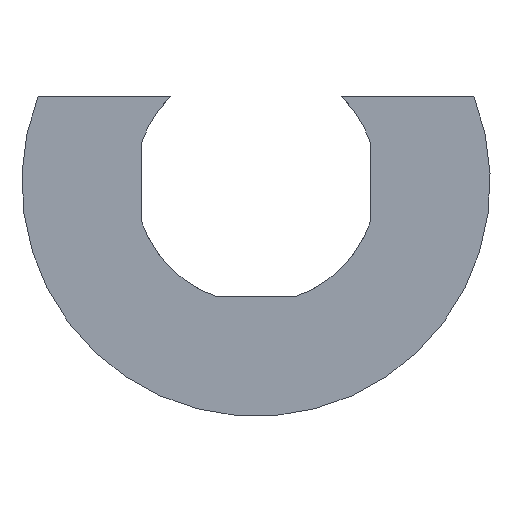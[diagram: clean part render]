
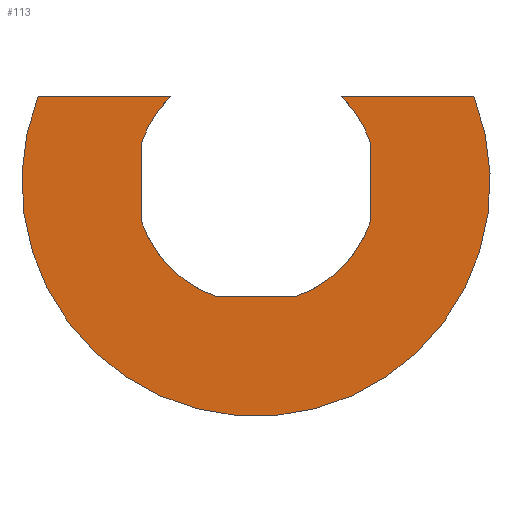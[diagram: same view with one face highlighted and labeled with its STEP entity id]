
A CAD part, front view. The second image highlights one B-rep face of the part: STEP entity #113.
In plain terms, the highlighted planar face has unit normal (0, -1, 0).
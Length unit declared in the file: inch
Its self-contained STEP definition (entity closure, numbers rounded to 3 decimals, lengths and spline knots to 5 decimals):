
#43 = EDGE_CURVE ( 'NONE', #423, #445, #149, .T. ) ;
#46 = EDGE_CURVE ( 'NONE', #447, #430, #778, .T. ) ;
#50 = EDGE_CURVE ( 'NONE', #438, #419, #141, .T. ) ;
#54 = EDGE_CURVE ( 'NONE', #419, #403, #821, .T. ) ;
#57 = EDGE_CURVE ( 'NONE', #418, #423, #824, .T. ) ;
#62 = EDGE_CURVE ( 'NONE', #447, #446, #145, .T. ) ;
#67 = EDGE_CURVE ( 'NONE', #446, #438, #838, .T. ) ;
#68 = EDGE_CURVE ( 'NONE', #418, #430, #143, .T. ) ;
#69 = EDGE_CURVE ( 'NONE', #405, #445, #840, .T. ) ;
#71 = EDGE_CURVE ( 'NONE', #403, #405, #168, .T. ) ;
#113 = ADVANCED_FACE ( 'NONE', ( #332 ), #987, .F. ) ;
#141 = CIRCLE ( 'NONE', #268, 0.60076 ) ;
#143 = CIRCLE ( 'NONE', #255, 0.60076 ) ;
#145 = CIRCLE ( 'NONE', #258, 0.60076 ) ;
#149 = CIRCLE ( 'NONE', #243, 1.16129 ) ;
#168 = CIRCLE ( 'NONE', #259, 0.60076 ) ;
#243 = AXIS2_PLACEMENT_3D ( 'NONE', #771, #768, #783 ) ;
#250 = VECTOR ( 'NONE', #859, 39.37008 ) ;
#255 = AXIS2_PLACEMENT_3D ( 'NONE', #846, #835, #832 ) ;
#256 = VECTOR ( 'NONE', #825, 39.37008 ) ;
#257 = VECTOR ( 'NONE', #806, 39.37008 ) ;
#258 = AXIS2_PLACEMENT_3D ( 'NONE', #815, #833, #850 ) ;
#259 = AXIS2_PLACEMENT_3D ( 'NONE', #851, #836, #853 ) ;
#260 = VECTOR ( 'NONE', #779, 39.37008 ) ;
#268 = AXIS2_PLACEMENT_3D ( 'NONE', #794, #787, #793 ) ;
#288 = VECTOR ( 'NONE', #852, 39.37008 ) ;
#310 = AXIS2_PLACEMENT_3D ( 'NONE', #990, #960, #963 ) ;
#332 = FACE_OUTER_BOUND ( 'NONE', #477, .T. ) ;
#403 = VERTEX_POINT ( 'NONE', #1159 ) ;
#405 = VERTEX_POINT ( 'NONE', #1160 ) ;
#418 = VERTEX_POINT ( 'NONE', #1179 ) ;
#419 = VERTEX_POINT ( 'NONE', #1184 ) ;
#423 = VERTEX_POINT ( 'NONE', #1183 ) ;
#430 = VERTEX_POINT ( 'NONE', #1098 ) ;
#438 = VERTEX_POINT ( 'NONE', #1097 ) ;
#445 = VERTEX_POINT ( 'NONE', #1048 ) ;
#446 = VERTEX_POINT ( 'NONE', #1050 ) ;
#447 = VERTEX_POINT ( 'NONE', #1033 ) ;
#477 = EDGE_LOOP ( 'NONE', ( #531, #543, #535, #525, #521, #522, #536, #542, #530, #519 ) ) ;
#519 = ORIENTED_EDGE ( 'NONE', *, *, #54, .T. ) ;
#521 = ORIENTED_EDGE ( 'NONE', *, *, #68, .T. ) ;
#522 = ORIENTED_EDGE ( 'NONE', *, *, #46, .F. ) ;
#525 = ORIENTED_EDGE ( 'NONE', *, *, #57, .F. ) ;
#530 = ORIENTED_EDGE ( 'NONE', *, *, #50, .T. ) ;
#531 = ORIENTED_EDGE ( 'NONE', *, *, #71, .T. ) ;
#535 = ORIENTED_EDGE ( 'NONE', *, *, #43, .F. ) ;
#536 = ORIENTED_EDGE ( 'NONE', *, *, #62, .T. ) ;
#542 = ORIENTED_EDGE ( 'NONE', *, *, #67, .T. ) ;
#543 = ORIENTED_EDGE ( 'NONE', *, *, #69, .T. ) ;
#768 = DIRECTION ( 'NONE',  ( 0., 1., 0. ) ) ;
#771 = CARTESIAN_POINT ( 'NONE',  ( -0.56759, 0., -0.19685 ) ) ;
#778 = LINE ( 'NONE', #786, #260 ) ;
#779 = DIRECTION ( 'NONE',  ( 0., 0., 1. ) ) ;
#783 = DIRECTION ( 'NONE',  ( 0., 0., 1. ) ) ;
#786 = CARTESIAN_POINT ( 'NONE',  ( 0., 0., 0. ) ) ;
#787 = DIRECTION ( 'NONE',  ( 0., 1., 0. ) ) ;
#793 = DIRECTION ( 'NONE',  ( 0., 0., 1. ) ) ;
#794 = CARTESIAN_POINT ( 'NONE',  ( -0.56759, 0., -0.19685 ) ) ;
#806 = DIRECTION ( 'NONE',  ( 0., 0., 1. ) ) ;
#807 = CARTESIAN_POINT ( 'NONE',  ( -1.13518, 0., 0. ) ) ;
#809 = CARTESIAN_POINT ( 'NONE',  ( 0., 0., 0.22795 ) ) ;
#815 = CARTESIAN_POINT ( 'NONE',  ( -0.56759, 0., -0.19685 ) ) ;
#821 = LINE ( 'NONE', #807, #257 ) ;
#824 = LINE ( 'NONE', #809, #256 ) ;
#825 = DIRECTION ( 'NONE',  ( 1., 0., 0. ) ) ;
#832 = DIRECTION ( 'NONE',  ( 0., 0., 1. ) ) ;
#833 = DIRECTION ( 'NONE',  ( 0., 1., 0. ) ) ;
#835 = DIRECTION ( 'NONE',  ( 0., 1., 0. ) ) ;
#836 = DIRECTION ( 'NONE',  ( 0., 1., 0. ) ) ;
#837 = CARTESIAN_POINT ( 'NONE',  ( 0., 0., 0.22795 ) ) ;
#838 = LINE ( 'NONE', #858, #250 ) ;
#840 = LINE ( 'NONE', #837, #288 ) ;
#846 = CARTESIAN_POINT ( 'NONE',  ( -0.56759, 0., -0.19685 ) ) ;
#850 = DIRECTION ( 'NONE',  ( 0., 0., 1. ) ) ;
#851 = CARTESIAN_POINT ( 'NONE',  ( -0.56759, 0., -0.19685 ) ) ;
#852 = DIRECTION ( 'NONE',  ( -1., 0., 0. ) ) ;
#853 = DIRECTION ( 'NONE',  ( 0., 0., 1. ) ) ;
#858 = CARTESIAN_POINT ( 'NONE',  ( 0., 0., -0.76444 ) ) ;
#859 = DIRECTION ( 'NONE',  ( -1., 0., 0. ) ) ;
#960 = DIRECTION ( 'NONE',  ( 0., 1., 0. ) ) ;
#963 = DIRECTION ( 'NONE',  ( 0., 0., 1. ) ) ;
#987 = PLANE ( 'NONE',  #310 ) ;
#990 = CARTESIAN_POINT ( 'NONE',  ( 0., 0., 0. ) ) ;
#1033 = CARTESIAN_POINT ( 'NONE',  ( 0., 0., -0.3937 ) ) ;
#1048 = CARTESIAN_POINT ( 'NONE',  ( -1.64839, 0., 0.22795 ) ) ;
#1050 = CARTESIAN_POINT ( 'NONE',  ( -0.37074, 0., -0.76444 ) ) ;
#1097 = CARTESIAN_POINT ( 'NONE',  ( -0.76444, 0., -0.76444 ) ) ;
#1098 = CARTESIAN_POINT ( 'NONE',  ( 0., 0., 0. ) ) ;
#1159 = CARTESIAN_POINT ( 'NONE',  ( -1.13518, 0., 0. ) ) ;
#1160 = CARTESIAN_POINT ( 'NONE',  ( -0.99239, 0., 0.22795 ) ) ;
#1179 = CARTESIAN_POINT ( 'NONE',  ( -0.14279, 0., 0.22795 ) ) ;
#1183 = CARTESIAN_POINT ( 'NONE',  ( 0.51322, 0., 0.22795 ) ) ;
#1184 = CARTESIAN_POINT ( 'NONE',  ( -1.13518, 0., -0.3937 ) ) ;
